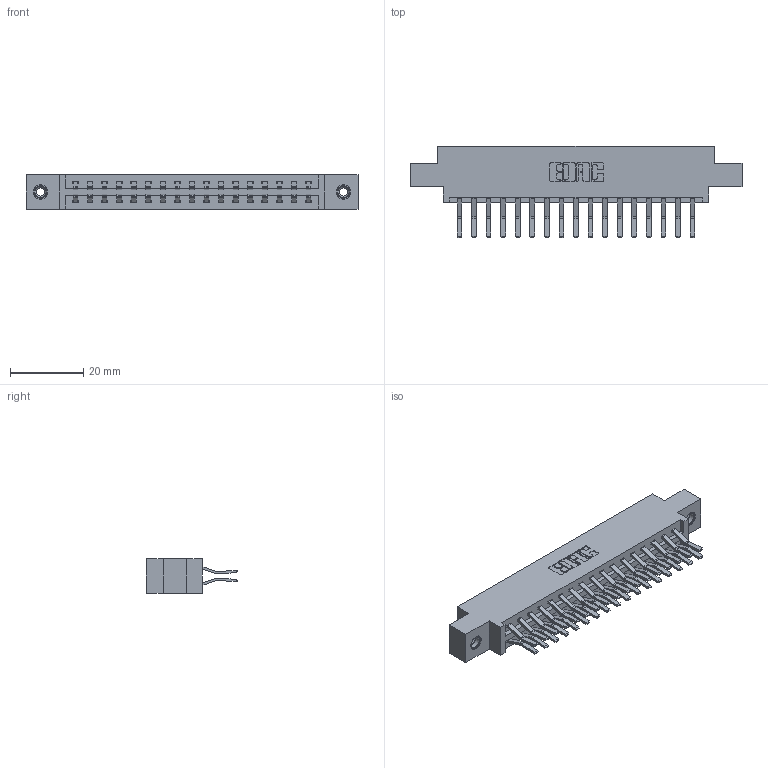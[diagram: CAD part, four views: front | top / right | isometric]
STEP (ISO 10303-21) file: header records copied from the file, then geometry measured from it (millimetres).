
FILE_DESCRIPTION (( 'STEP AP203' ), '1' );
FILE_NAME ('387-034-560-808.STEP', '2019-10-17T18:33:49', ( '' ), ( '' ), 'SwSTEP 2.0', 'SolidWorks 2016', '' );
FILE_SCHEMA (( 'CONFIG_CONTROL_DESIGN' ));
Length unit declared in the file: inch
Products named in the file (4): 345-250-001_345-250-003-102; 345-292-001_560 Tail; 387-034-560-808; 337 Part_0.170 Offset - 0.156 Dia-TI
Assembly tree (37 placements, depth 2):
  387-034-560-808
    337 Part_0.170 Offset - 0.156 Dia-TI
    345-292-001_560 Tail  x34
    345-250-001_345-250-003-102  x2
Bounding box: 90.37 x 24.78 x 9.4 mm (x, y, z)
Volume: 9290.3 mm3; surface area: 11036.6 mm2
Topology: 37 solids, 37 shells, 2082 faces, 6137 edges, 4038 vertices
Faces by surface type: plane 1398, cylinder 668, cone 12, torus 4
Entity records: 17820 total; most frequent: CARTESIAN_POINT 3005, ORIENTED_EDGE 2934, DIRECTION 2637, EDGE_CURVE 1467, LINE 1315, VECTOR 1315, VERTEX_POINT 972, AXIS2_PLACEMENT_3D 661
